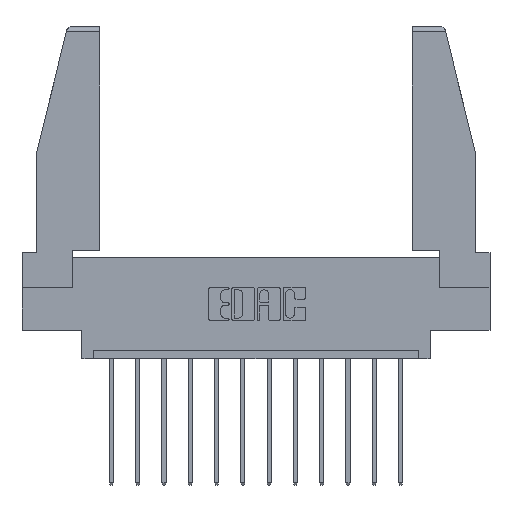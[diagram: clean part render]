
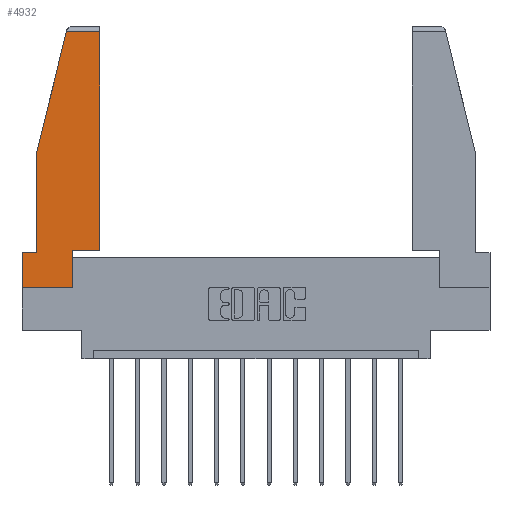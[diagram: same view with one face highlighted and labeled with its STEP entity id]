
A CAD part, top view. The second image highlights one B-rep face of the part: STEP entity #4932.
In plain terms, the highlighted planar face has unit normal (0, 0, 1).
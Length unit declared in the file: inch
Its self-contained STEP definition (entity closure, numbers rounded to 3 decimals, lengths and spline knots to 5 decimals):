
#351 = CARTESIAN_POINT ( 'NONE',  ( 0.2636, 1.52, 0. ) ) ;
#659 = CARTESIAN_POINT ( 'NONE',  ( 0.461, 1.52, 0. ) ) ;
#686 = VECTOR ( 'NONE', #2565, 39.37008 ) ;
#728 = VERTEX_POINT ( 'NONE', #6157 ) ;
#1004 = VECTOR ( 'NONE', #13537, 39.37008 ) ;
#1142 = LINE ( 'NONE', #12115, #6576 ) ;
#1236 = ORIENTED_EDGE ( 'NONE', *, *, #13597, .T. ) ;
#1584 = FACE_OUTER_BOUND ( 'NONE', #10760, .T. ) ;
#1868 = ORIENTED_EDGE ( 'NONE', *, *, #10757, .T. ) ;
#2090 = DIRECTION ( 'NONE',  ( 0., 1., 0. ) ) ;
#2276 = EDGE_CURVE ( 'NONE', #12562, #14789, #10214, .T. ) ;
#2369 = DIRECTION ( 'NONE',  ( -0.239, -0.971, 0. ) ) ;
#2386 = CARTESIAN_POINT ( 'NONE',  ( 0.086, 0.21, 0. ) ) ;
#2565 = DIRECTION ( 'NONE',  ( 0., -1., 0. ) ) ;
#2677 = EDGE_CURVE ( 'NONE', #4772, #11782, #14840, .T. ) ;
#2738 = VECTOR ( 'NONE', #2090, 39.37008 ) ;
#2817 = DIRECTION ( 'NONE',  ( 1., 0., 0. ) ) ;
#3347 = ORIENTED_EDGE ( 'NONE', *, *, #11024, .T. ) ;
#3740 = DIRECTION ( 'NONE',  ( 0., 1., 0. ) ) ;
#4158 = CARTESIAN_POINT ( 'NONE',  ( 0., 0., 0. ) ) ;
#4373 = LINE ( 'NONE', #12314, #1004 ) ;
#4632 = ORIENTED_EDGE ( 'NONE', *, *, #13952, .T. ) ;
#4772 = VERTEX_POINT ( 'NONE', #5802 ) ;
#4932 = ADVANCED_FACE ( 'NONE', ( #1584 ), #11923, .T. ) ;
#5078 = VECTOR ( 'NONE', #2817, 39.37008 ) ;
#5476 = VERTEX_POINT ( 'NONE', #5629 ) ;
#5629 = CARTESIAN_POINT ( 'NONE',  ( 0.297, 0., 0. ) ) ;
#5802 = CARTESIAN_POINT ( 'NONE',  ( 0.086, 0.8, 0. ) ) ;
#6157 = CARTESIAN_POINT ( 'NONE',  ( 0.297, 0.223, 0. ) ) ;
#6576 = VECTOR ( 'NONE', #2369, 39.37008 ) ;
#6663 = AXIS2_PLACEMENT_3D ( 'NONE', #8399, #13182, #7120 ) ;
#6860 = CARTESIAN_POINT ( 'NONE',  ( 0., 1.52, 0. ) ) ;
#7120 = DIRECTION ( 'NONE',  ( 1., 0., 0. ) ) ;
#7306 = CARTESIAN_POINT ( 'NONE',  ( 0., 0., 0. ) ) ;
#8108 = VERTEX_POINT ( 'NONE', #659 ) ;
#8399 = CARTESIAN_POINT ( 'NONE',  ( 0., 0., 0. ) ) ;
#8629 = LINE ( 'NONE', #10868, #11955 ) ;
#8654 = CARTESIAN_POINT ( 'NONE',  ( 0., 0.21, 0. ) ) ;
#8850 = ORIENTED_EDGE ( 'NONE', *, *, #11389, .T. ) ;
#9471 = VECTOR ( 'NONE', #13745, 39.37008 ) ;
#9824 = ORIENTED_EDGE ( 'NONE', *, *, #2677, .T. ) ;
#9834 = EDGE_CURVE ( 'NONE', #11782, #12562, #4373, .T. ) ;
#10070 = VERTEX_POINT ( 'NONE', #351 ) ;
#10214 = LINE ( 'NONE', #13842, #9471 ) ;
#10464 = ORIENTED_EDGE ( 'NONE', *, *, #9834, .T. ) ;
#10694 = DIRECTION ( 'NONE',  ( 1., 0., 0. ) ) ;
#10757 = EDGE_CURVE ( 'NONE', #11860, #8108, #8629, .T. ) ;
#10760 = EDGE_LOOP ( 'NONE', ( #1868, #15330, #3347, #9824, #10464, #14665, #8850, #1236, #4632 ) ) ;
#10868 = CARTESIAN_POINT ( 'NONE',  ( 0.461, 0.223, 0. ) ) ;
#11004 = CARTESIAN_POINT ( 'NONE',  ( 0.086, 0.8, 0. ) ) ;
#11024 = EDGE_CURVE ( 'NONE', #10070, #4772, #1142, .T. ) ;
#11389 = EDGE_CURVE ( 'NONE', #14789, #5476, #13617, .T. ) ;
#11586 = CARTESIAN_POINT ( 'NONE',  ( 0.297, 0., 0. ) ) ;
#11670 = EDGE_CURVE ( 'NONE', #8108, #10070, #15185, .T. ) ;
#11782 = VERTEX_POINT ( 'NONE', #2386 ) ;
#11860 = VERTEX_POINT ( 'NONE', #13239 ) ;
#11923 = PLANE ( 'NONE',  #6663 ) ;
#11928 = CARTESIAN_POINT ( 'NONE',  ( 0.297, 0.223, 0. ) ) ;
#11955 = VECTOR ( 'NONE', #3740, 39.37008 ) ;
#12115 = CARTESIAN_POINT ( 'NONE',  ( 0.271, 1.55, 0. ) ) ;
#12314 = CARTESIAN_POINT ( 'NONE',  ( 0., 0.21, 0. ) ) ;
#12562 = VERTEX_POINT ( 'NONE', #8654 ) ;
#12931 = VECTOR ( 'NONE', #10694, 39.37008 ) ;
#13182 = DIRECTION ( 'NONE',  ( 0., 0., 1. ) ) ;
#13239 = CARTESIAN_POINT ( 'NONE',  ( 0.461, 0.223, 0. ) ) ;
#13537 = DIRECTION ( 'NONE',  ( -1., 0., 0. ) ) ;
#13597 = EDGE_CURVE ( 'NONE', #5476, #728, #14635, .T. ) ;
#13617 = LINE ( 'NONE', #4158, #5078 ) ;
#13745 = DIRECTION ( 'NONE',  ( 0., -1., 0. ) ) ;
#13842 = CARTESIAN_POINT ( 'NONE',  ( 0., 0.21, 0. ) ) ;
#13952 = EDGE_CURVE ( 'NONE', #728, #11860, #14432, .T. ) ;
#14432 = LINE ( 'NONE', #11928, #12931 ) ;
#14635 = LINE ( 'NONE', #11586, #2738 ) ;
#14665 = ORIENTED_EDGE ( 'NONE', *, *, #2276, .T. ) ;
#14789 = VERTEX_POINT ( 'NONE', #7306 ) ;
#14840 = LINE ( 'NONE', #11004, #686 ) ;
#15185 = LINE ( 'NONE', #6860, #15348 ) ;
#15209 = DIRECTION ( 'NONE',  ( -1., 0., 0. ) ) ;
#15330 = ORIENTED_EDGE ( 'NONE', *, *, #11670, .T. ) ;
#15348 = VECTOR ( 'NONE', #15209, 39.37008 ) ;
